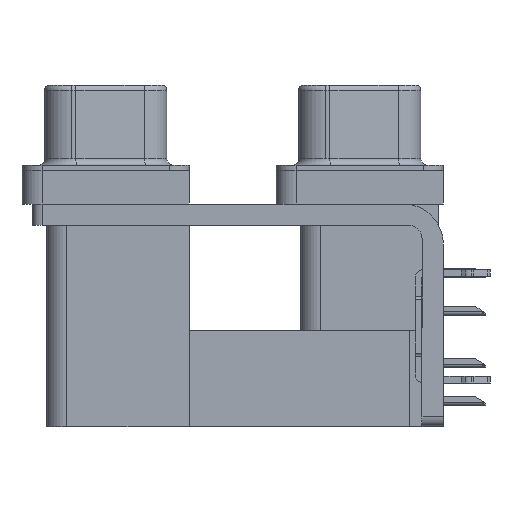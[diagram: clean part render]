
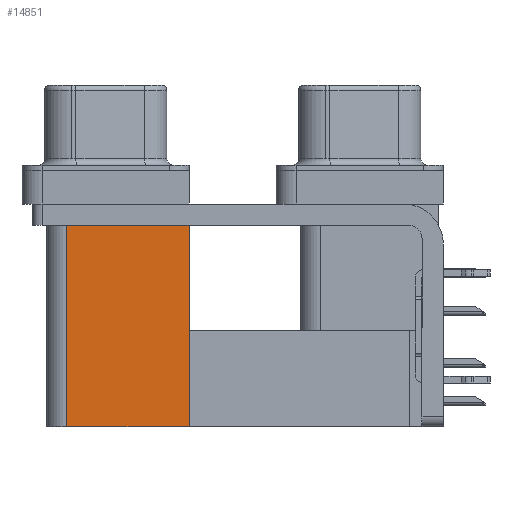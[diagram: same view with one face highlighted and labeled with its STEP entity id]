
A CAD part, left-side view. The second image highlights one B-rep face of the part: STEP entity #14851.
In plain terms, the highlighted planar face has unit normal (-1, 0, 0).
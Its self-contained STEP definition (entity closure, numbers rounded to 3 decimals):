
#1161 = PLANE ( 'NONE',  #21285 ) ;
#1228 = VECTOR ( 'NONE', #8599, 1000. ) ;
#2795 = CARTESIAN_POINT ( 'NONE',  ( 3.765, 12.775, -2.5 ) ) ;
#3901 = LINE ( 'NONE', #5814, #20604 ) ;
#5814 = CARTESIAN_POINT ( 'NONE',  ( 3.765, 12.775, -19.2 ) ) ;
#6323 = DIRECTION ( 'NONE',  ( 0., 0., 1. ) ) ;
#8599 = DIRECTION ( 'NONE',  ( 0., 1., 0. ) ) ;
#10299 = EDGE_CURVE ( 'NONE', #27750, #28260, #3901, .T. ) ;
#10869 = EDGE_LOOP ( 'NONE', ( #33712, #13779, #27344, #23388 ) ) ;
#11176 = CARTESIAN_POINT ( 'NONE',  ( 3.765, 12.775, -19.2 ) ) ;
#11894 = CARTESIAN_POINT ( 'NONE',  ( 3.765, 21.975, -19.2 ) ) ;
#12172 = VECTOR ( 'NONE', #13277, 1000. ) ;
#13277 = DIRECTION ( 'NONE',  ( 0., 1., 0. ) ) ;
#13779 = ORIENTED_EDGE ( 'NONE', *, *, #33012, .F. ) ;
#13916 = LINE ( 'NONE', #11176, #1228 ) ;
#14121 = VERTEX_POINT ( 'NONE', #11894 ) ;
#14851 = ADVANCED_FACE ( 'NONE', ( #27460 ), #1161, .F. ) ;
#16988 = DIRECTION ( 'NONE',  ( 0., 0., -1. ) ) ;
#18452 = LINE ( 'NONE', #2795, #12172 ) ;
#18460 = CARTESIAN_POINT ( 'NONE',  ( 3.765, 12.775, -2.5 ) ) ;
#20356 = CARTESIAN_POINT ( 'NONE',  ( 3.765, 21.975, -19.2 ) ) ;
#20604 = VECTOR ( 'NONE', #6323, 1000. ) ;
#21285 = AXIS2_PLACEMENT_3D ( 'NONE', #32123, #29541, #16988 ) ;
#21810 = VERTEX_POINT ( 'NONE', #23991 ) ;
#23388 = ORIENTED_EDGE ( 'NONE', *, *, #10299, .T. ) ;
#23991 = CARTESIAN_POINT ( 'NONE',  ( 3.765, 21.975, -2.5 ) ) ;
#25320 = LINE ( 'NONE', #20356, #28341 ) ;
#27097 = EDGE_CURVE ( 'NONE', #28260, #21810, #18452, .T. ) ;
#27344 = ORIENTED_EDGE ( 'NONE', *, *, #27535, .F. ) ;
#27460 = FACE_OUTER_BOUND ( 'NONE', #10869, .T. ) ;
#27535 = EDGE_CURVE ( 'NONE', #27750, #14121, #13916, .T. ) ;
#27750 = VERTEX_POINT ( 'NONE', #28311 ) ;
#28089 = DIRECTION ( 'NONE',  ( 0., 0., 1. ) ) ;
#28260 = VERTEX_POINT ( 'NONE', #18460 ) ;
#28311 = CARTESIAN_POINT ( 'NONE',  ( 3.765, 12.775, -19.2 ) ) ;
#28341 = VECTOR ( 'NONE', #28089, 1000. ) ;
#29541 = DIRECTION ( 'NONE',  ( 1., 0., 0. ) ) ;
#32123 = CARTESIAN_POINT ( 'NONE',  ( 3.765, 12.775, -19.2 ) ) ;
#33012 = EDGE_CURVE ( 'NONE', #14121, #21810, #25320, .T. ) ;
#33712 = ORIENTED_EDGE ( 'NONE', *, *, #27097, .T. ) ;
